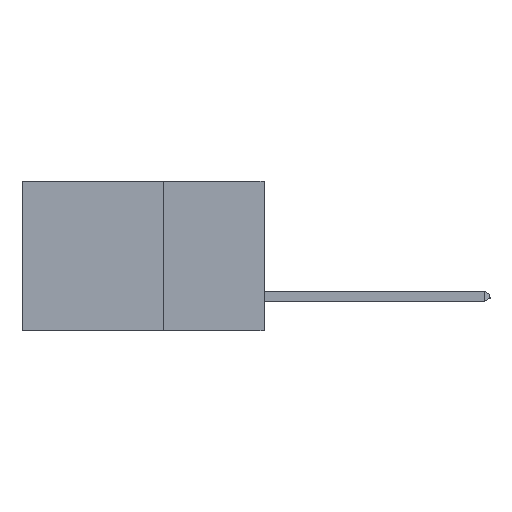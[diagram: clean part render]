
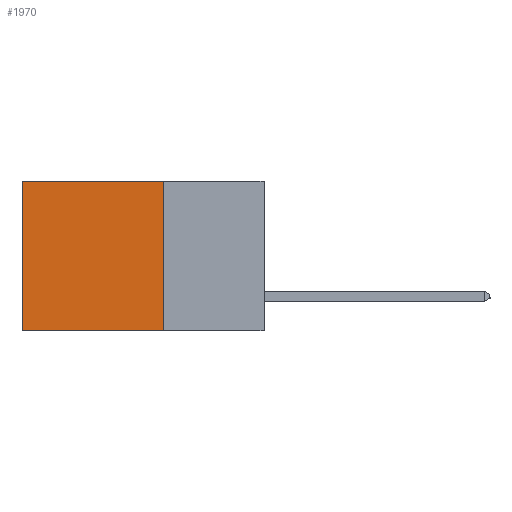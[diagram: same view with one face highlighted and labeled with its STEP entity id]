
A CAD part, left-side view. The second image highlights one B-rep face of the part: STEP entity #1970.
In plain terms, the highlighted planar face has unit normal (-1, 0, 0).
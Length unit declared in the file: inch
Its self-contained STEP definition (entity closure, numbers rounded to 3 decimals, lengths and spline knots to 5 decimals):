
#360 = VECTOR ( 'NONE', #7416, 39.37008 ) ;
#440 = CARTESIAN_POINT ( 'NONE',  ( 0.298, 0.25, 0. ) ) ;
#1111 = EDGE_CURVE ( 'NONE', #6046, #4587, #10098, .T. ) ;
#1567 = CARTESIAN_POINT ( 'NONE',  ( 0.298, 0.25, 0. ) ) ;
#1970 = ADVANCED_FACE ( 'NONE', ( #7244 ), #4660, .F. ) ;
#2423 = ORIENTED_EDGE ( 'NONE', *, *, #6646, .T. ) ;
#2762 = ORIENTED_EDGE ( 'NONE', *, *, #5938, .T. ) ;
#3499 = DIRECTION ( 'NONE',  ( 0., 1., 0. ) ) ;
#3904 = CARTESIAN_POINT ( 'NONE',  ( 0.298, 0.25, -0.37 ) ) ;
#3928 = CARTESIAN_POINT ( 'NONE',  ( 0.298, 0.25, 0. ) ) ;
#3972 = CARTESIAN_POINT ( 'NONE',  ( 0.298, 0.6, -0.37 ) ) ;
#4229 = CARTESIAN_POINT ( 'NONE',  ( 0.298, 0.25, 0. ) ) ;
#4587 = VERTEX_POINT ( 'NONE', #3904 ) ;
#4660 = PLANE ( 'NONE',  #7967 ) ;
#5092 = ORIENTED_EDGE ( 'NONE', *, *, #5714, .F. ) ;
#5292 = DIRECTION ( 'NONE',  ( 1., 0., 0. ) ) ;
#5310 = LINE ( 'NONE', #11834, #10060 ) ;
#5489 = CARTESIAN_POINT ( 'NONE',  ( 0.298, 0.6, 0. ) ) ;
#5714 = EDGE_CURVE ( 'NONE', #4587, #10576, #8473, .T. ) ;
#5938 = EDGE_CURVE ( 'NONE', #6046, #8389, #6093, .T. ) ;
#6046 = VERTEX_POINT ( 'NONE', #1567 ) ;
#6093 = LINE ( 'NONE', #3928, #10837 ) ;
#6646 = EDGE_CURVE ( 'NONE', #8389, #10576, #5310, .T. ) ;
#7244 = FACE_OUTER_BOUND ( 'NONE', #8525, .T. ) ;
#7274 = VECTOR ( 'NONE', #9331, 39.37008 ) ;
#7404 = DIRECTION ( 'NONE',  ( 0., 0., -1. ) ) ;
#7416 = DIRECTION ( 'NONE',  ( 0., 1., 0. ) ) ;
#7636 = ORIENTED_EDGE ( 'NONE', *, *, #1111, .F. ) ;
#7915 = CARTESIAN_POINT ( 'NONE',  ( 0.298, 0.25, -0.37 ) ) ;
#7967 = AXIS2_PLACEMENT_3D ( 'NONE', #440, #5292, #7404 ) ;
#8389 = VERTEX_POINT ( 'NONE', #5489 ) ;
#8473 = LINE ( 'NONE', #7915, #360 ) ;
#8525 = EDGE_LOOP ( 'NONE', ( #2423, #5092, #7636, #2762 ) ) ;
#9331 = DIRECTION ( 'NONE',  ( 0., 0., -1. ) ) ;
#10060 = VECTOR ( 'NONE', #12737, 39.37008 ) ;
#10098 = LINE ( 'NONE', #4229, #7274 ) ;
#10576 = VERTEX_POINT ( 'NONE', #3972 ) ;
#10837 = VECTOR ( 'NONE', #3499, 39.37008 ) ;
#11834 = CARTESIAN_POINT ( 'NONE',  ( 0.298, 0.6, 0. ) ) ;
#12737 = DIRECTION ( 'NONE',  ( 0., 0., -1. ) ) ;
